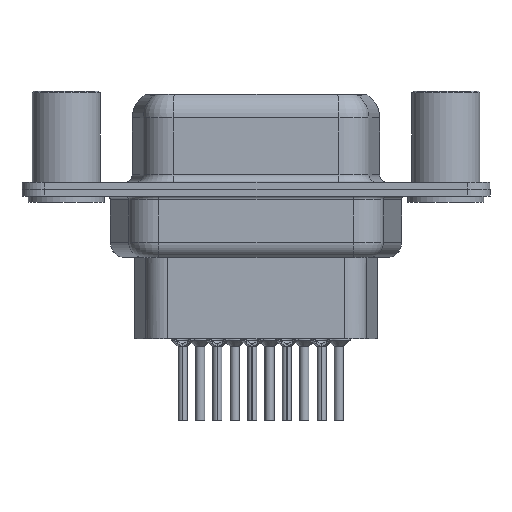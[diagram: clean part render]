
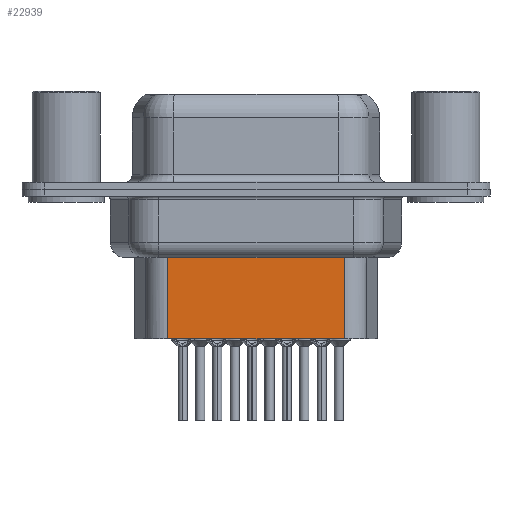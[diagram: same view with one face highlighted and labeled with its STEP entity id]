
A CAD part, front view. The second image highlights one B-rep face of the part: STEP entity #22939.
In plain terms, the highlighted planar face has unit normal (0, -1, 0).
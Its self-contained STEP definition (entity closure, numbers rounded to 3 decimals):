
#517 = EDGE_CURVE ( 'NONE', #25101, #19621, #8692, .T. ) ;
#565 = CARTESIAN_POINT ( 'NONE',  ( 6.454, -3.5, -4.097 ) ) ;
#1331 = CARTESIAN_POINT ( 'NONE',  ( 6.701, -3.5, -9.85 ) ) ;
#2668 = VECTOR ( 'NONE', #22666, 1000. ) ;
#3236 = PLANE ( 'NONE',  #18786 ) ;
#5109 = LINE ( 'NONE', #20422, #28285 ) ;
#5280 = ORIENTED_EDGE ( 'NONE', *, *, #19662, .T. ) ;
#6263 = ORIENTED_EDGE ( 'NONE', *, *, #23922, .F. ) ;
#8692 = LINE ( 'NONE', #565, #2668 ) ;
#9690 = DIRECTION ( 'NONE',  ( 0., 0., -1. ) ) ;
#10547 = EDGE_CURVE ( 'NONE', #25101, #21624, #28735, .T. ) ;
#11850 = VECTOR ( 'NONE', #14234, 1000. ) ;
#12279 = DIRECTION ( 'NONE',  ( 1., 0., 0. ) ) ;
#14234 = DIRECTION ( 'NONE',  ( 0., 0., -1. ) ) ;
#16261 = CARTESIAN_POINT ( 'NONE',  ( 6.701, -3.5, -4.097 ) ) ;
#16330 = CARTESIAN_POINT ( 'NONE',  ( 18.289, -3.5, -3.1 ) ) ;
#17648 = EDGE_LOOP ( 'NONE', ( #18685, #25486, #5280, #6263 ) ) ;
#18685 = ORIENTED_EDGE ( 'NONE', *, *, #10547, .F. ) ;
#18786 = AXIS2_PLACEMENT_3D ( 'NONE', #21188, #25707, #12279 ) ;
#19621 = VERTEX_POINT ( 'NONE', #16261 ) ;
#19662 = EDGE_CURVE ( 'NONE', #19621, #23061, #29028, .T. ) ;
#20422 = CARTESIAN_POINT ( 'NONE',  ( 6.701, -3.5, -9.85 ) ) ;
#21188 = CARTESIAN_POINT ( 'NONE',  ( 6.701, -3.5, -3.1 ) ) ;
#21624 = VERTEX_POINT ( 'NONE', #26881 ) ;
#22666 = DIRECTION ( 'NONE',  ( -1., 0., 0. ) ) ;
#22681 = DIRECTION ( 'NONE',  ( -1., 0., 0. ) ) ;
#22750 = VECTOR ( 'NONE', #9690, 1000. ) ;
#22939 = ADVANCED_FACE ( 'NONE', ( #27969 ), #3236, .T. ) ;
#23061 = VERTEX_POINT ( 'NONE', #1331 ) ;
#23922 = EDGE_CURVE ( 'NONE', #21624, #23061, #5109, .T. ) ;
#25101 = VERTEX_POINT ( 'NONE', #28156 ) ;
#25486 = ORIENTED_EDGE ( 'NONE', *, *, #517, .T. ) ;
#25707 = DIRECTION ( 'NONE',  ( 0., -1., 0. ) ) ;
#26881 = CARTESIAN_POINT ( 'NONE',  ( 18.289, -3.5, -9.85 ) ) ;
#27646 = CARTESIAN_POINT ( 'NONE',  ( 6.701, -3.5, -3.1 ) ) ;
#27969 = FACE_OUTER_BOUND ( 'NONE', #17648, .T. ) ;
#28156 = CARTESIAN_POINT ( 'NONE',  ( 18.289, -3.5, -4.097 ) ) ;
#28285 = VECTOR ( 'NONE', #22681, 1000. ) ;
#28735 = LINE ( 'NONE', #16330, #22750 ) ;
#29028 = LINE ( 'NONE', #27646, #11850 ) ;
